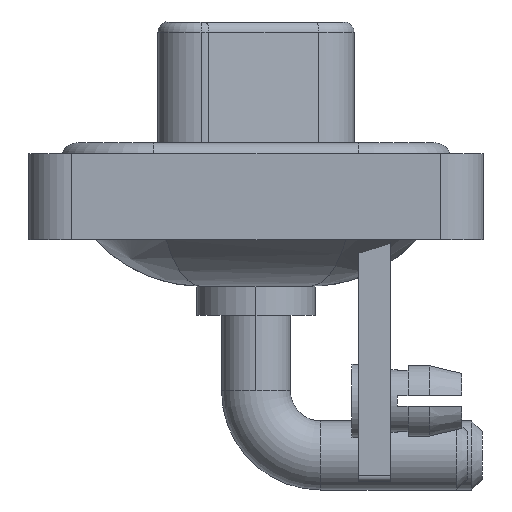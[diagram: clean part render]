
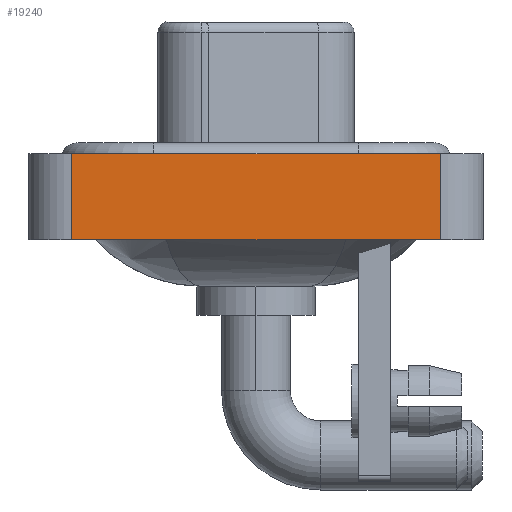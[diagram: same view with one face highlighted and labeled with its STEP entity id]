
A CAD part, left-side view. The second image highlights one B-rep face of the part: STEP entity #19240.
In plain terms, the highlighted planar face has unit normal (-1, 0, 0).
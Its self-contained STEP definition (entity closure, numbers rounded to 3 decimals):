
#143 = DIRECTION ( 'NONE',  ( 0., 0., 1. ) ) ;
#380 = EDGE_CURVE ( 'NONE', #3923, #7388, #6950, .T. ) ;
#596 = CARTESIAN_POINT ( 'NONE',  ( -7.3, 8.55, -3.6 ) ) ;
#613 = CARTESIAN_POINT ( 'NONE',  ( -7.3, -8.55, -3.6 ) ) ;
#2001 = CARTESIAN_POINT ( 'NONE',  ( -7.3, -8.55, 0.4 ) ) ;
#3758 = CARTESIAN_POINT ( 'NONE',  ( -7.3, -8.55, -3.6 ) ) ;
#3923 = VERTEX_POINT ( 'NONE', #16826 ) ;
#4090 = CARTESIAN_POINT ( 'NONE',  ( -7.3, 8.55, -3.6 ) ) ;
#5331 = DIRECTION ( 'NONE',  ( 0., 0., 1. ) ) ;
#5414 = VERTEX_POINT ( 'NONE', #596 ) ;
#5647 = DIRECTION ( 'NONE',  ( 0., -1., 0. ) ) ;
#6804 = AXIS2_PLACEMENT_3D ( 'NONE', #6884, #17064, #5331 ) ;
#6884 = CARTESIAN_POINT ( 'NONE',  ( -7.3, -8.55, -3.6 ) ) ;
#6886 = VECTOR ( 'NONE', #143, 1000. ) ;
#6950 = LINE ( 'NONE', #3758, #6886 ) ;
#7386 = LINE ( 'NONE', #4090, #19451 ) ;
#7388 = VERTEX_POINT ( 'NONE', #7484 ) ;
#7484 = CARTESIAN_POINT ( 'NONE',  ( -7.3, -8.55, 0.4 ) ) ;
#8519 = PLANE ( 'NONE',  #6804 ) ;
#9075 = EDGE_CURVE ( 'NONE', #17872, #7388, #13373, .T. ) ;
#10170 = FACE_OUTER_BOUND ( 'NONE', #21496, .T. ) ;
#12104 = DIRECTION ( 'NONE',  ( 0., 0., 1. ) ) ;
#12621 = ORIENTED_EDGE ( 'NONE', *, *, #9075, .F. ) ;
#13222 = VECTOR ( 'NONE', #20389, 1000. ) ;
#13373 = LINE ( 'NONE', #2001, #13222 ) ;
#15919 = EDGE_CURVE ( 'NONE', #5414, #17872, #7386, .T. ) ;
#16335 = ORIENTED_EDGE ( 'NONE', *, *, #380, .T. ) ;
#16586 = VECTOR ( 'NONE', #5647, 1000. ) ;
#16826 = CARTESIAN_POINT ( 'NONE',  ( -7.3, -8.55, -3.6 ) ) ;
#17064 = DIRECTION ( 'NONE',  ( -1., 0., 0. ) ) ;
#17274 = LINE ( 'NONE', #613, #16586 ) ;
#17872 = VERTEX_POINT ( 'NONE', #20343 ) ;
#19240 = ADVANCED_FACE ( 'NONE', ( #10170 ), #8519, .T. ) ;
#19406 = EDGE_CURVE ( 'NONE', #5414, #3923, #17274, .T. ) ;
#19451 = VECTOR ( 'NONE', #12104, 1000. ) ;
#20124 = ORIENTED_EDGE ( 'NONE', *, *, #15919, .F. ) ;
#20343 = CARTESIAN_POINT ( 'NONE',  ( -7.3, 8.55, 0.4 ) ) ;
#20389 = DIRECTION ( 'NONE',  ( 0., -1., 0. ) ) ;
#20517 = ORIENTED_EDGE ( 'NONE', *, *, #19406, .T. ) ;
#21496 = EDGE_LOOP ( 'NONE', ( #16335, #12621, #20124, #20517 ) ) ;
